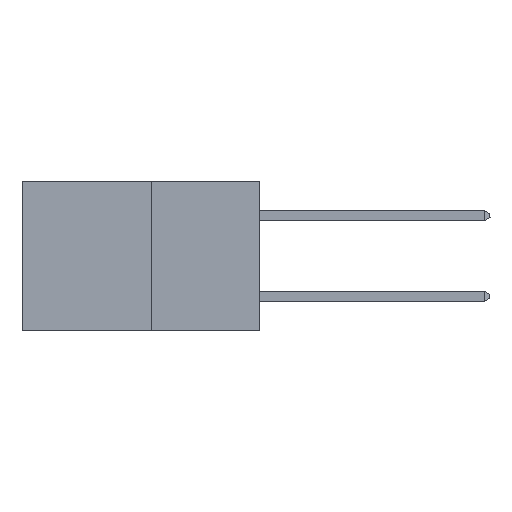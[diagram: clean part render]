
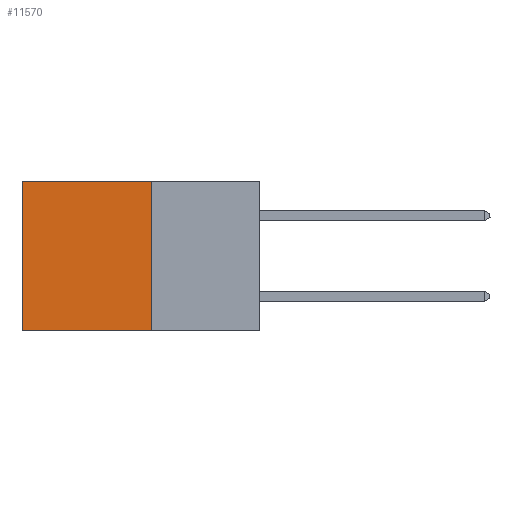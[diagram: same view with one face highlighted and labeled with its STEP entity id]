
A CAD part, left-side view. The second image highlights one B-rep face of the part: STEP entity #11570.
In plain terms, the highlighted planar face has unit normal (-1, 0, 0).
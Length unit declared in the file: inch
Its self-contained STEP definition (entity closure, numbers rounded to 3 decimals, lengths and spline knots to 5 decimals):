
#396 = FACE_OUTER_BOUND ( 'NONE', #2281, .T. ) ;
#545 = EDGE_CURVE ( 'NONE', #1705, #4673, #11287, .T. ) ;
#1467 = CARTESIAN_POINT ( 'NONE',  ( 0.277, 0.59, 0. ) ) ;
#1705 = VERTEX_POINT ( 'NONE', #8532 ) ;
#2281 = EDGE_LOOP ( 'NONE', ( #3941, #5114, #4837, #6120 ) ) ;
#2288 = DIRECTION ( 'NONE',  ( 0., 1., 0. ) ) ;
#2763 = VECTOR ( 'NONE', #2288, 39.37008 ) ;
#3006 = DIRECTION ( 'NONE',  ( 0., 1., 0. ) ) ;
#3176 = CARTESIAN_POINT ( 'NONE',  ( 0.277, 0.59, -0.37 ) ) ;
#3516 = EDGE_CURVE ( 'NONE', #4297, #8974, #10734, .T. ) ;
#3941 = ORIENTED_EDGE ( 'NONE', *, *, #11734, .T. ) ;
#4045 = DIRECTION ( 'NONE',  ( 1., 0., 0. ) ) ;
#4180 = CARTESIAN_POINT ( 'NONE',  ( 0.277, 0.27, -0.37 ) ) ;
#4273 = DIRECTION ( 'NONE',  ( 0., 0., -1. ) ) ;
#4297 = VERTEX_POINT ( 'NONE', #13132 ) ;
#4647 = VECTOR ( 'NONE', #9552, 39.37008 ) ;
#4673 = VERTEX_POINT ( 'NONE', #3176 ) ;
#4837 = ORIENTED_EDGE ( 'NONE', *, *, #11662, .F. ) ;
#5114 = ORIENTED_EDGE ( 'NONE', *, *, #545, .F. ) ;
#5975 = CARTESIAN_POINT ( 'NONE',  ( 0.277, 0.27, -0.37 ) ) ;
#6120 = ORIENTED_EDGE ( 'NONE', *, *, #3516, .T. ) ;
#6873 = VECTOR ( 'NONE', #4273, 39.37008 ) ;
#7284 = PLANE ( 'NONE',  #10225 ) ;
#7593 = VECTOR ( 'NONE', #3006, 39.37008 ) ;
#8215 = LINE ( 'NONE', #4180, #4647 ) ;
#8532 = CARTESIAN_POINT ( 'NONE',  ( 0.277, 0.27, -0.37 ) ) ;
#8974 = VERTEX_POINT ( 'NONE', #1467 ) ;
#9552 = DIRECTION ( 'NONE',  ( 0., 0., -1. ) ) ;
#10225 = AXIS2_PLACEMENT_3D ( 'NONE', #10478, #4045, #11497 ) ;
#10478 = CARTESIAN_POINT ( 'NONE',  ( 0.277, 0.27, -0.37 ) ) ;
#10500 = CARTESIAN_POINT ( 'NONE',  ( 0.277, 0.27, 0. ) ) ;
#10734 = LINE ( 'NONE', #10500, #7593 ) ;
#11287 = LINE ( 'NONE', #5975, #2763 ) ;
#11497 = DIRECTION ( 'NONE',  ( 0., 0., -1. ) ) ;
#11570 = ADVANCED_FACE ( 'NONE', ( #396 ), #7284, .F. ) ;
#11662 = EDGE_CURVE ( 'NONE', #4297, #1705, #8215, .T. ) ;
#11734 = EDGE_CURVE ( 'NONE', #8974, #4673, #12504, .T. ) ;
#11736 = CARTESIAN_POINT ( 'NONE',  ( 0.277, 0.59, -0.37 ) ) ;
#12504 = LINE ( 'NONE', #11736, #6873 ) ;
#13132 = CARTESIAN_POINT ( 'NONE',  ( 0.277, 0.27, 0. ) ) ;
